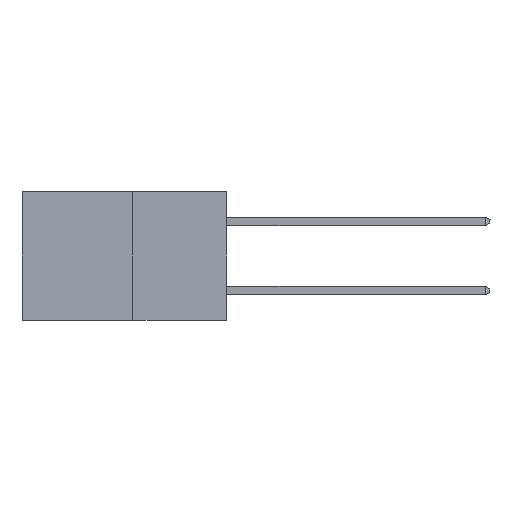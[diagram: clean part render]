
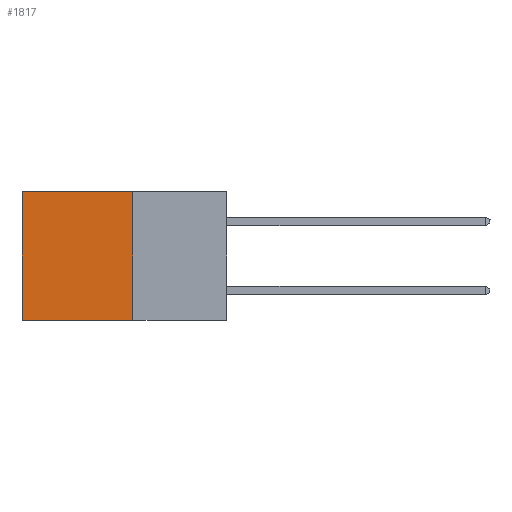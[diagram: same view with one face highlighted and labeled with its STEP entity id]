
A CAD part, left-side view. The second image highlights one B-rep face of the part: STEP entity #1817.
In plain terms, the highlighted planar face has unit normal (-1, 0, 0).
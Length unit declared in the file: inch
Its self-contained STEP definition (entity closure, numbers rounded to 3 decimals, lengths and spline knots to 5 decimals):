
#10 = CARTESIAN_POINT ( 'NONE',  ( 0.277, 0.27, 0. ) ) ;
#179 = EDGE_CURVE ( 'NONE', #17252, #10109, #8144, .T. ) ;
#790 = CARTESIAN_POINT ( 'NONE',  ( 0.277, 0.59, -0.37 ) ) ;
#800 = CARTESIAN_POINT ( 'NONE',  ( 0.277, 0.27, 0. ) ) ;
#1672 = DIRECTION ( 'NONE',  ( 0., 1., 0. ) ) ;
#1817 = ADVANCED_FACE ( 'NONE', ( #13865 ), #16352, .F. ) ;
#1929 = ORIENTED_EDGE ( 'NONE', *, *, #8448, .F. ) ;
#2383 = ORIENTED_EDGE ( 'NONE', *, *, #11466, .T. ) ;
#2561 = CARTESIAN_POINT ( 'NONE',  ( 0.277, 0.27, -0.37 ) ) ;
#4205 = CARTESIAN_POINT ( 'NONE',  ( 0.277, 0.27, -0.37 ) ) ;
#4362 = CARTESIAN_POINT ( 'NONE',  ( 0.277, 0.59, 0. ) ) ;
#4603 = VECTOR ( 'NONE', #14199, 39.37008 ) ;
#4804 = CARTESIAN_POINT ( 'NONE',  ( 0.277, 0.59, -0.37 ) ) ;
#5308 = CARTESIAN_POINT ( 'NONE',  ( 0.277, 0.27, -0.37 ) ) ;
#5584 = LINE ( 'NONE', #10, #17689 ) ;
#5906 = DIRECTION ( 'NONE',  ( 0., 0., -1. ) ) ;
#8144 = LINE ( 'NONE', #790, #15815 ) ;
#8277 = AXIS2_PLACEMENT_3D ( 'NONE', #20339, #18161, #18091 ) ;
#8448 = EDGE_CURVE ( 'NONE', #15877, #18919, #19777, .T. ) ;
#9243 = DIRECTION ( 'NONE',  ( 0., 0., -1. ) ) ;
#10109 = VERTEX_POINT ( 'NONE', #4804 ) ;
#11120 = VECTOR ( 'NONE', #5906, 39.37008 ) ;
#11466 = EDGE_CURVE ( 'NONE', #15877, #17252, #5584, .T. ) ;
#11870 = ORIENTED_EDGE ( 'NONE', *, *, #179, .T. ) ;
#13413 = LINE ( 'NONE', #2561, #4603 ) ;
#13865 = FACE_OUTER_BOUND ( 'NONE', #17028, .T. ) ;
#14199 = DIRECTION ( 'NONE',  ( 0., 1., 0. ) ) ;
#14683 = EDGE_CURVE ( 'NONE', #18919, #10109, #13413, .T. ) ;
#15815 = VECTOR ( 'NONE', #9243, 39.37008 ) ;
#15877 = VERTEX_POINT ( 'NONE', #800 ) ;
#16352 = PLANE ( 'NONE',  #8277 ) ;
#16655 = ORIENTED_EDGE ( 'NONE', *, *, #14683, .F. ) ;
#17028 = EDGE_LOOP ( 'NONE', ( #11870, #16655, #1929, #2383 ) ) ;
#17252 = VERTEX_POINT ( 'NONE', #4362 ) ;
#17689 = VECTOR ( 'NONE', #1672, 39.37008 ) ;
#18091 = DIRECTION ( 'NONE',  ( 0., 0., -1. ) ) ;
#18161 = DIRECTION ( 'NONE',  ( 1., 0., 0. ) ) ;
#18919 = VERTEX_POINT ( 'NONE', #5308 ) ;
#19777 = LINE ( 'NONE', #4205, #11120 ) ;
#20339 = CARTESIAN_POINT ( 'NONE',  ( 0.277, 0.27, -0.37 ) ) ;
